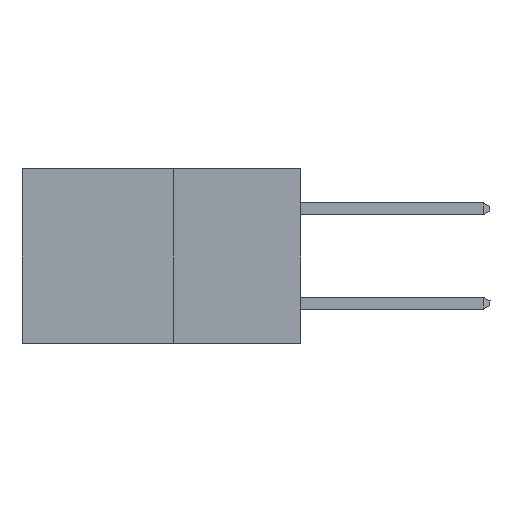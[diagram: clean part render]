
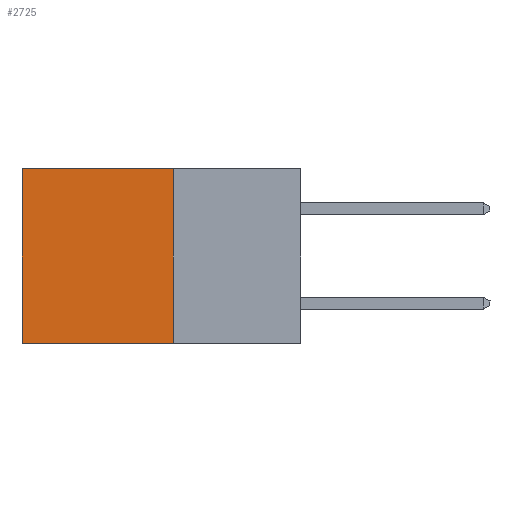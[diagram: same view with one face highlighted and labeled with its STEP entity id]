
A CAD part, left-side view. The second image highlights one B-rep face of the part: STEP entity #2725.
In plain terms, the highlighted planar face has unit normal (-1, 0, 0).
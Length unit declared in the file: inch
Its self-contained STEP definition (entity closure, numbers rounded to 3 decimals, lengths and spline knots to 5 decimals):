
#1228 = EDGE_CURVE ( 'NONE', #14135, #18204, #18325, .T. ) ;
#1988 = LINE ( 'NONE', #27484, #13029 ) ;
#2053 = EDGE_CURVE ( 'NONE', #24980, #14135, #3884, .T. ) ;
#2225 = DIRECTION ( 'NONE',  ( 0., 0., -1. ) ) ;
#2725 = ADVANCED_FACE ( 'NONE', ( #20286 ), #15265, .F. ) ;
#3204 = VECTOR ( 'NONE', #26467, 39.37008 ) ;
#3884 = LINE ( 'NONE', #22164, #3204 ) ;
#5064 = EDGE_CURVE ( 'NONE', #24980, #10134, #1988, .T. ) ;
#5686 = EDGE_CURVE ( 'NONE', #10134, #18204, #14025, .T. ) ;
#5967 = CARTESIAN_POINT ( 'NONE',  ( 0.277, 0.27, -0.37 ) ) ;
#6419 = CARTESIAN_POINT ( 'NONE',  ( 0.277, 0.27, -0.37 ) ) ;
#8061 = CARTESIAN_POINT ( 'NONE',  ( 0.277, 0.59, 0. ) ) ;
#8845 = VECTOR ( 'NONE', #25418, 39.37008 ) ;
#10122 = ORIENTED_EDGE ( 'NONE', *, *, #5686, .T. ) ;
#10134 = VERTEX_POINT ( 'NONE', #8061 ) ;
#11053 = DIRECTION ( 'NONE',  ( 1., 0., 0. ) ) ;
#12062 = ORIENTED_EDGE ( 'NONE', *, *, #1228, .F. ) ;
#12542 = VECTOR ( 'NONE', #12809, 39.37008 ) ;
#12809 = DIRECTION ( 'NONE',  ( 0., 1., 0. ) ) ;
#13029 = VECTOR ( 'NONE', #17863, 39.37008 ) ;
#14025 = LINE ( 'NONE', #25454, #8845 ) ;
#14135 = VERTEX_POINT ( 'NONE', #20614 ) ;
#14375 = EDGE_LOOP ( 'NONE', ( #10122, #12062, #26223, #19727 ) ) ;
#15265 = PLANE ( 'NONE',  #20129 ) ;
#17687 = CARTESIAN_POINT ( 'NONE',  ( 0.277, 0.59, -0.37 ) ) ;
#17863 = DIRECTION ( 'NONE',  ( 0., 1., 0. ) ) ;
#18204 = VERTEX_POINT ( 'NONE', #17687 ) ;
#18325 = LINE ( 'NONE', #6419, #12542 ) ;
#19069 = CARTESIAN_POINT ( 'NONE',  ( 0.277, 0.27, 0. ) ) ;
#19727 = ORIENTED_EDGE ( 'NONE', *, *, #5064, .T. ) ;
#20129 = AXIS2_PLACEMENT_3D ( 'NONE', #5967, #11053, #2225 ) ;
#20286 = FACE_OUTER_BOUND ( 'NONE', #14375, .T. ) ;
#20614 = CARTESIAN_POINT ( 'NONE',  ( 0.277, 0.27, -0.37 ) ) ;
#22164 = CARTESIAN_POINT ( 'NONE',  ( 0.277, 0.27, -0.37 ) ) ;
#24980 = VERTEX_POINT ( 'NONE', #19069 ) ;
#25418 = DIRECTION ( 'NONE',  ( 0., 0., -1. ) ) ;
#25454 = CARTESIAN_POINT ( 'NONE',  ( 0.277, 0.59, -0.37 ) ) ;
#26223 = ORIENTED_EDGE ( 'NONE', *, *, #2053, .F. ) ;
#26467 = DIRECTION ( 'NONE',  ( 0., 0., -1. ) ) ;
#27484 = CARTESIAN_POINT ( 'NONE',  ( 0.277, 0.27, 0. ) ) ;
